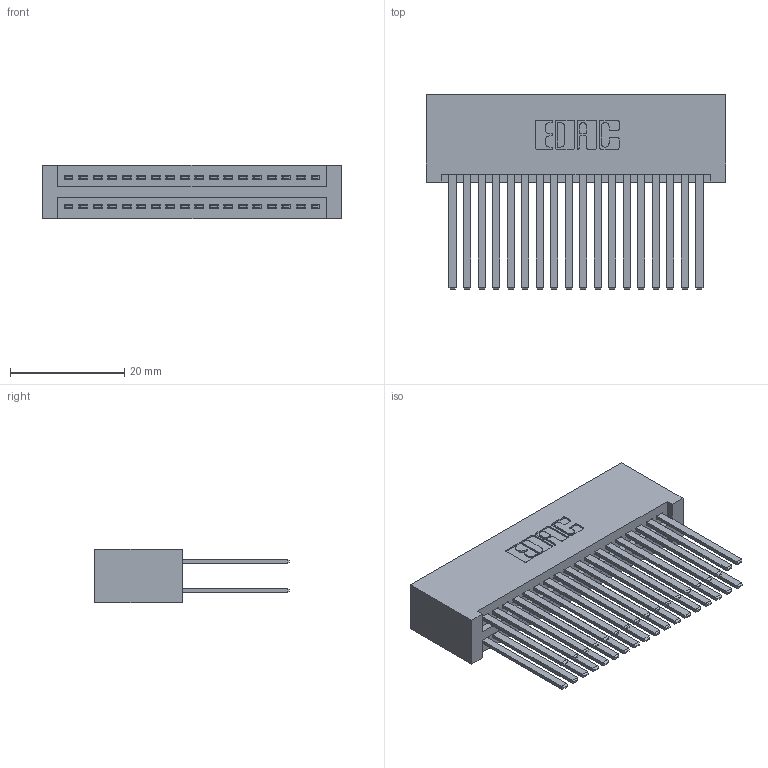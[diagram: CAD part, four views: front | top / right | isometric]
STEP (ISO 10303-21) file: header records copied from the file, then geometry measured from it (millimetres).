
FILE_DESCRIPTION (( 'STEP AP203' ), '1' );
FILE_NAME ('345-036-544-201.STEP', '2018-08-29T23:37:35', ( '' ), ( '' ), 'SwSTEP 2.0', 'SolidWorks 2016', '' );
FILE_SCHEMA (( 'CONFIG_CONTROL_DESIGN' ));
Length unit declared in the file: inch
Products named in the file (3): 345-036-544-201; 345 Part_No Mounting Lugs; 345-292-001_345-293-144
Assembly tree (37 placements, depth 2):
  345-036-544-201
    345 Part_No Mounting Lugs
    345-292-001_345-293-144  x36
Bounding box: 52.32 x 33.96 x 9.4 mm (x, y, z)
Volume: 5980.6 mm3; surface area: 10157.9 mm2
Topology: 37 solids, 37 shells, 1702 faces, 5033 edges, 3306 vertices
Faces by surface type: plane 1120, cylinder 582
Entity records: 16893 total; most frequent: CARTESIAN_POINT 2852, ORIENTED_EDGE 2786, DIRECTION 2537, EDGE_CURVE 1393, LINE 1201, VECTOR 1201, VERTEX_POINT 926, AXIS2_PLACEMENT_3D 668
